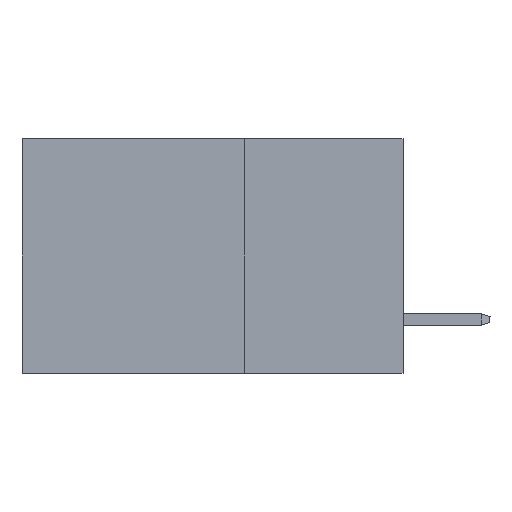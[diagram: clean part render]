
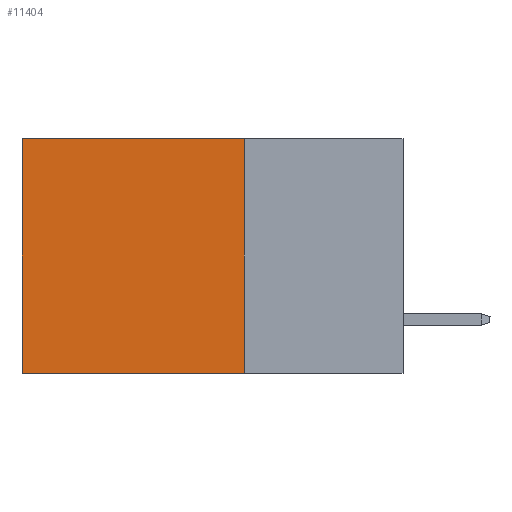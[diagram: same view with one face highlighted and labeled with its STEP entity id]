
A CAD part, left-side view. The second image highlights one B-rep face of the part: STEP entity #11404.
In plain terms, the highlighted planar face has unit normal (-1, 0, 0).
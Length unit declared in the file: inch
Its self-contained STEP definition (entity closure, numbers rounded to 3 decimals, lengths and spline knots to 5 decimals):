
#1410 = CARTESIAN_POINT ( 'NONE',  ( 0.2875, 0.6, -0.37 ) ) ;
#3222 = ORIENTED_EDGE ( 'NONE', *, *, #5331, .T. ) ;
#3298 = CARTESIAN_POINT ( 'NONE',  ( 0.2875, 0.25, 0. ) ) ;
#3371 = VERTEX_POINT ( 'NONE', #22596 ) ;
#3787 = FACE_OUTER_BOUND ( 'NONE', #28482, .T. ) ;
#3806 = VERTEX_POINT ( 'NONE', #1410 ) ;
#5060 = LINE ( 'NONE', #9947, #5950 ) ;
#5331 = EDGE_CURVE ( 'NONE', #3371, #13268, #23313, .T. ) ;
#5950 = VECTOR ( 'NONE', #11891, 39.37008 ) ;
#6241 = CARTESIAN_POINT ( 'NONE',  ( 0.2875, 0.6, 0. ) ) ;
#7355 = DIRECTION ( 'NONE',  ( 0., 0., -1. ) ) ;
#8503 = EDGE_CURVE ( 'NONE', #13268, #3806, #14962, .T. ) ;
#9368 = VECTOR ( 'NONE', #30776, 39.37008 ) ;
#9947 = CARTESIAN_POINT ( 'NONE',  ( 0.2875, 0.25, -0.37 ) ) ;
#10529 = ORIENTED_EDGE ( 'NONE', *, *, #25569, .F. ) ;
#11404 = ADVANCED_FACE ( 'NONE', ( #3787 ), #21360, .F. ) ;
#11508 = VECTOR ( 'NONE', #13176, 39.37008 ) ;
#11891 = DIRECTION ( 'NONE',  ( 0., 1., 0. ) ) ;
#13176 = DIRECTION ( 'NONE',  ( 0., 1., 0. ) ) ;
#13268 = VERTEX_POINT ( 'NONE', #6241 ) ;
#14962 = LINE ( 'NONE', #29599, #25204 ) ;
#15779 = CARTESIAN_POINT ( 'NONE',  ( 0.2875, 0.25, 0. ) ) ;
#17219 = VERTEX_POINT ( 'NONE', #24946 ) ;
#20757 = CARTESIAN_POINT ( 'NONE',  ( 0.2875, 0.25, 0. ) ) ;
#21360 = PLANE ( 'NONE',  #25709 ) ;
#22596 = CARTESIAN_POINT ( 'NONE',  ( 0.2875, 0.25, 0. ) ) ;
#23205 = LINE ( 'NONE', #20757, #9368 ) ;
#23313 = LINE ( 'NONE', #15779, #11508 ) ;
#23478 = DIRECTION ( 'NONE',  ( 0., 0., -1. ) ) ;
#24946 = CARTESIAN_POINT ( 'NONE',  ( 0.2875, 0.25, -0.37 ) ) ;
#25204 = VECTOR ( 'NONE', #7355, 39.37008 ) ;
#25569 = EDGE_CURVE ( 'NONE', #3371, #17219, #23205, .T. ) ;
#25709 = AXIS2_PLACEMENT_3D ( 'NONE', #3298, #25798, #23478 ) ;
#25798 = DIRECTION ( 'NONE',  ( 1., 0., 0. ) ) ;
#25829 = ORIENTED_EDGE ( 'NONE', *, *, #26109, .F. ) ;
#26109 = EDGE_CURVE ( 'NONE', #17219, #3806, #5060, .T. ) ;
#28078 = ORIENTED_EDGE ( 'NONE', *, *, #8503, .T. ) ;
#28482 = EDGE_LOOP ( 'NONE', ( #28078, #25829, #10529, #3222 ) ) ;
#29599 = CARTESIAN_POINT ( 'NONE',  ( 0.2875, 0.6, 0. ) ) ;
#30776 = DIRECTION ( 'NONE',  ( 0., 0., -1. ) ) ;
